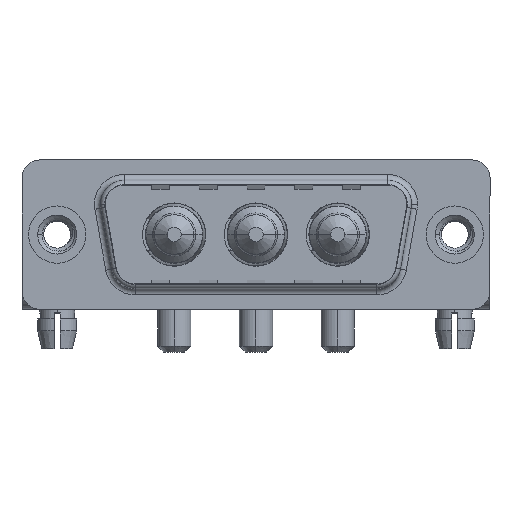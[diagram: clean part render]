
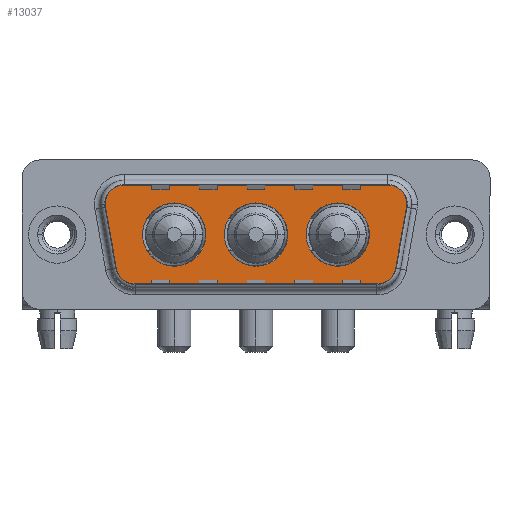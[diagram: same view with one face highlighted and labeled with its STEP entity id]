
A CAD part, top view. The second image highlights one B-rep face of the part: STEP entity #13037.
In plain terms, the highlighted planar face has unit normal (0, 0, 1).
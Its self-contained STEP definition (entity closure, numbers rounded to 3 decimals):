
#108 = VECTOR ( 'NONE', #428, 1000. ) ;
#158 = DIRECTION ( 'NONE',  ( 0., 0., 1. ) ) ;
#182 = DIRECTION ( 'NONE',  ( 0., 0., 1. ) ) ;
#191 = LINE ( 'NONE', #11911, #4817 ) ;
#214 = EDGE_LOOP ( 'NONE', ( #3924, #3839 ) ) ;
#377 = AXIS2_PLACEMENT_3D ( 'NONE', #4697, #10625, #3537 ) ;
#426 = ORIENTED_EDGE ( 'NONE', *, *, #8593, .T. ) ;
#428 = DIRECTION ( 'NONE',  ( 1., 0., 0. ) ) ;
#639 = CARTESIAN_POINT ( 'NONE',  ( 29.859, 2.553, 0. ) ) ;
#1091 = CARTESIAN_POINT ( 'NONE',  ( 23.5, 0., 0. ) ) ;
#1105 = EDGE_CURVE ( 'NONE', #3271, #3332, #7468, .T. ) ;
#1198 = CARTESIAN_POINT ( 'NONE',  ( 6.434, -4.9, 0. ) ) ;
#1291 = CIRCLE ( 'NONE', #2038, 2.65 ) ;
#1300 = VERTEX_POINT ( 'NONE', #15241 ) ;
#1457 = EDGE_CURVE ( 'NONE', #7131, #4285, #4489, .T. ) ;
#1855 = DIRECTION ( 'NONE',  ( -1., 0., 0. ) ) ;
#2038 = AXIS2_PLACEMENT_3D ( 'NONE', #11796, #158, #10727 ) ;
#2148 = PLANE ( 'NONE',  #10729 ) ;
#2660 = CARTESIAN_POINT ( 'NONE',  ( 4.464, -3.247, 0. ) ) ;
#2708 = CARTESIAN_POINT ( 'NONE',  ( 14., 0., 0. ) ) ;
#2712 = ORIENTED_EDGE ( 'NONE', *, *, #1105, .T. ) ;
#2839 = DIRECTION ( 'NONE',  ( 1., 0., 0. ) ) ;
#2892 = AXIS2_PLACEMENT_3D ( 'NONE', #12554, #13554, #1855 ) ;
#2941 = DIRECTION ( 'NONE',  ( 0., 0., 1. ) ) ;
#2997 = ORIENTED_EDGE ( 'NONE', *, *, #1457, .F. ) ;
#3063 = EDGE_CURVE ( 'NONE', #7741, #11018, #11179, .T. ) ;
#3137 = CARTESIAN_POINT ( 'NONE',  ( 6.434, -4.9, 0. ) ) ;
#3167 = CARTESIAN_POINT ( 'NONE',  ( 23.5, 0., 0. ) ) ;
#3230 = DIRECTION ( 'NONE',  ( 1., 0., 0. ) ) ;
#3271 = VERTEX_POINT ( 'NONE', #1198 ) ;
#3278 = CIRCLE ( 'NONE', #3787, 2. ) ;
#3294 = FACE_BOUND ( 'NONE', #214, .T. ) ;
#3332 = VERTEX_POINT ( 'NONE', #12827 ) ;
#3537 = DIRECTION ( 'NONE',  ( -1., 0., 0. ) ) ;
#3613 = ORIENTED_EDGE ( 'NONE', *, *, #4195, .T. ) ;
#3621 = CIRCLE ( 'NONE', #2892, 2. ) ;
#3776 = DIRECTION ( 'NONE',  ( 1., 0., 0. ) ) ;
#3787 = AXIS2_PLACEMENT_3D ( 'NONE', #8560, #9641, #3776 ) ;
#3839 = ORIENTED_EDGE ( 'NONE', *, *, #14009, .F. ) ;
#3924 = ORIENTED_EDGE ( 'NONE', *, *, #3063, .F. ) ;
#3953 = ORIENTED_EDGE ( 'NONE', *, *, #6250, .F. ) ;
#3984 = EDGE_CURVE ( 'NONE', #14954, #5148, #3621, .T. ) ;
#4163 = CARTESIAN_POINT ( 'NONE',  ( 7.15, 0., 0. ) ) ;
#4195 = EDGE_CURVE ( 'NONE', #11799, #14954, #8035, .T. ) ;
#4198 = ORIENTED_EDGE ( 'NONE', *, *, #6032, .T. ) ;
#4285 = VERTEX_POINT ( 'NONE', #12009 ) ;
#4361 = AXIS2_PLACEMENT_3D ( 'NONE', #12782, #8108, #8400 ) ;
#4489 = CIRCLE ( 'NONE', #7964, 2.65 ) ;
#4661 = DIRECTION ( 'NONE',  ( 0.174, 0.985, 0. ) ) ;
#4686 = DIRECTION ( 'NONE',  ( 0., 0., 1. ) ) ;
#4697 = CARTESIAN_POINT ( 'NONE',  ( 27.889, 2.9, 0. ) ) ;
#4764 = FACE_BOUND ( 'NONE', #10945, .T. ) ;
#4817 = VECTOR ( 'NONE', #6148, 1000. ) ;
#5148 = VERTEX_POINT ( 'NONE', #15151 ) ;
#5508 = CARTESIAN_POINT ( 'NONE',  ( 20.85, 0., 0. ) ) ;
#5581 = CIRCLE ( 'NONE', #10491, 2.65 ) ;
#5820 = DIRECTION ( 'NONE',  ( 0., 0., 1. ) ) ;
#5856 = FACE_BOUND ( 'NONE', #11167, .T. ) ;
#5889 = DIRECTION ( 'NONE',  ( 1., 0., 0. ) ) ;
#6032 = EDGE_CURVE ( 'NONE', #1300, #10187, #8946, .T. ) ;
#6148 = DIRECTION ( 'NONE',  ( 0.174, -0.985, 0. ) ) ;
#6250 = EDGE_CURVE ( 'NONE', #4285, #7131, #1291, .T. ) ;
#6390 = CARTESIAN_POINT ( 'NONE',  ( 5.411, 4.9, 0. ) ) ;
#6705 = VERTEX_POINT ( 'NONE', #2660 ) ;
#6746 = AXIS2_PLACEMENT_3D ( 'NONE', #13466, #13701, #2839 ) ;
#6758 = ORIENTED_EDGE ( 'NONE', *, *, #7805, .T. ) ;
#6893 = LINE ( 'NONE', #12895, #7948 ) ;
#7131 = VERTEX_POINT ( 'NONE', #2708 ) ;
#7134 = CARTESIAN_POINT ( 'NONE',  ( 16.65, 0., 0. ) ) ;
#7356 = CIRCLE ( 'NONE', #8089, 2.65 ) ;
#7468 = LINE ( 'NONE', #3137, #108 ) ;
#7560 = LINE ( 'NONE', #6390, #8062 ) ;
#7652 = DIRECTION ( 'NONE',  ( -1., 0., 0. ) ) ;
#7741 = VERTEX_POINT ( 'NONE', #8934 ) ;
#7805 = EDGE_CURVE ( 'NONE', #13552, #11799, #6893, .T. ) ;
#7948 = VECTOR ( 'NONE', #4661, 1000. ) ;
#7964 = AXIS2_PLACEMENT_3D ( 'NONE', #7134, #182, #9458 ) ;
#8035 = CIRCLE ( 'NONE', #377, 2. ) ;
#8050 = CARTESIAN_POINT ( 'NONE',  ( 5.411, 2.9, 0. ) ) ;
#8062 = VECTOR ( 'NONE', #8478, 1000. ) ;
#8089 = AXIS2_PLACEMENT_3D ( 'NONE', #1091, #5820, #15058 ) ;
#8108 = DIRECTION ( 'NONE',  ( 0., 0., 1. ) ) ;
#8400 = DIRECTION ( 'NONE',  ( 1., 0., 0. ) ) ;
#8478 = DIRECTION ( 'NONE',  ( -1., 0., 0. ) ) ;
#8560 = CARTESIAN_POINT ( 'NONE',  ( 26.866, -2.9, 0. ) ) ;
#8593 = EDGE_CURVE ( 'NONE', #6705, #3271, #11409, .T. ) ;
#8870 = EDGE_CURVE ( 'NONE', #3332, #13552, #3278, .T. ) ;
#8934 = CARTESIAN_POINT ( 'NONE',  ( 12.45, 0., 0. ) ) ;
#8946 = CIRCLE ( 'NONE', #15070, 2. ) ;
#9046 = ORIENTED_EDGE ( 'NONE', *, *, #11195, .T. ) ;
#9051 = VERTEX_POINT ( 'NONE', #14948 ) ;
#9068 = ORIENTED_EDGE ( 'NONE', *, *, #15098, .F. ) ;
#9126 = DIRECTION ( 'NONE',  ( 0., 0., 1. ) ) ;
#9458 = DIRECTION ( 'NONE',  ( 1., 0., 0. ) ) ;
#9568 = ORIENTED_EDGE ( 'NONE', *, *, #3984, .T. ) ;
#9641 = DIRECTION ( 'NONE',  ( 0., 0., 1. ) ) ;
#10187 = VERTEX_POINT ( 'NONE', #14210 ) ;
#10382 = CARTESIAN_POINT ( 'NONE',  ( 26.866, -2.9, 0. ) ) ;
#10491 = AXIS2_PLACEMENT_3D ( 'NONE', #3167, #9126, #3230 ) ;
#10538 = FACE_OUTER_BOUND ( 'NONE', #12880, .T. ) ;
#10591 = CARTESIAN_POINT ( 'NONE',  ( 29.889, 2.9, 0. ) ) ;
#10625 = DIRECTION ( 'NONE',  ( 0., 0., 1. ) ) ;
#10727 = DIRECTION ( 'NONE',  ( 1., 0., 0. ) ) ;
#10729 = AXIS2_PLACEMENT_3D ( 'NONE', #10382, #4686, #14080 ) ;
#10945 = EDGE_LOOP ( 'NONE', ( #9068, #11931 ) ) ;
#11018 = VERTEX_POINT ( 'NONE', #4163 ) ;
#11167 = EDGE_LOOP ( 'NONE', ( #3953, #2997 ) ) ;
#11179 = CIRCLE ( 'NONE', #6746, 2.65 ) ;
#11195 = EDGE_CURVE ( 'NONE', #10187, #6705, #191, .T. ) ;
#11409 = CIRCLE ( 'NONE', #15104, 2. ) ;
#11652 = DIRECTION ( 'NONE',  ( 0., 0., 1. ) ) ;
#11796 = CARTESIAN_POINT ( 'NONE',  ( 16.65, 0., 0. ) ) ;
#11799 = VERTEX_POINT ( 'NONE', #639 ) ;
#11911 = CARTESIAN_POINT ( 'NONE',  ( 3.441, 2.553, 0. ) ) ;
#11914 = VERTEX_POINT ( 'NONE', #5508 ) ;
#11931 = ORIENTED_EDGE ( 'NONE', *, *, #12490, .F. ) ;
#12009 = CARTESIAN_POINT ( 'NONE',  ( 19.3, 0., 0. ) ) ;
#12490 = EDGE_CURVE ( 'NONE', #11914, #9051, #5581, .T. ) ;
#12554 = CARTESIAN_POINT ( 'NONE',  ( 27.889, 2.9, 0. ) ) ;
#12782 = CARTESIAN_POINT ( 'NONE',  ( 9.8, 0., 0. ) ) ;
#12811 = EDGE_CURVE ( 'NONE', #5148, #1300, #7560, .T. ) ;
#12827 = CARTESIAN_POINT ( 'NONE',  ( 26.866, -4.9, 0. ) ) ;
#12880 = EDGE_LOOP ( 'NONE', ( #13943, #6758, #3613, #9568, #14063, #4198, #9046, #426, #2712 ) ) ;
#12895 = CARTESIAN_POINT ( 'NONE',  ( 29.859, 2.553, 0. ) ) ;
#13037 = ADVANCED_FACE ( 'NONE', ( #5856, #4764, #3294, #10538 ), #2148, .T. ) ;
#13466 = CARTESIAN_POINT ( 'NONE',  ( 9.8, 0., 0. ) ) ;
#13489 = CARTESIAN_POINT ( 'NONE',  ( 6.434, -2.9, 0. ) ) ;
#13552 = VERTEX_POINT ( 'NONE', #14354 ) ;
#13554 = DIRECTION ( 'NONE',  ( 0., 0., 1. ) ) ;
#13701 = DIRECTION ( 'NONE',  ( 0., 0., 1. ) ) ;
#13943 = ORIENTED_EDGE ( 'NONE', *, *, #8870, .T. ) ;
#14009 = EDGE_CURVE ( 'NONE', #11018, #7741, #14192, .T. ) ;
#14063 = ORIENTED_EDGE ( 'NONE', *, *, #12811, .T. ) ;
#14080 = DIRECTION ( 'NONE',  ( 1., 0., 0. ) ) ;
#14192 = CIRCLE ( 'NONE', #4361, 2.65 ) ;
#14210 = CARTESIAN_POINT ( 'NONE',  ( 3.441, 2.553, 0. ) ) ;
#14354 = CARTESIAN_POINT ( 'NONE',  ( 28.836, -3.247, 0. ) ) ;
#14948 = CARTESIAN_POINT ( 'NONE',  ( 26.15, 0., 0. ) ) ;
#14954 = VERTEX_POINT ( 'NONE', #10591 ) ;
#15058 = DIRECTION ( 'NONE',  ( 1., 0., 0. ) ) ;
#15070 = AXIS2_PLACEMENT_3D ( 'NONE', #8050, #11652, #5889 ) ;
#15098 = EDGE_CURVE ( 'NONE', #9051, #11914, #7356, .T. ) ;
#15104 = AXIS2_PLACEMENT_3D ( 'NONE', #13489, #2941, #7652 ) ;
#15151 = CARTESIAN_POINT ( 'NONE',  ( 27.889, 4.9, 0. ) ) ;
#15241 = CARTESIAN_POINT ( 'NONE',  ( 5.411, 4.9, 0. ) ) ;
